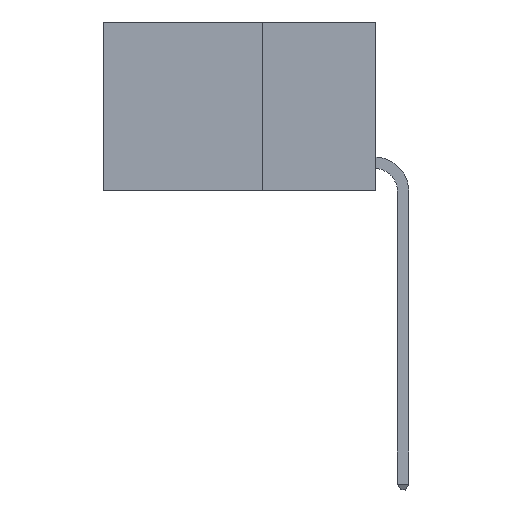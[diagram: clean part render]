
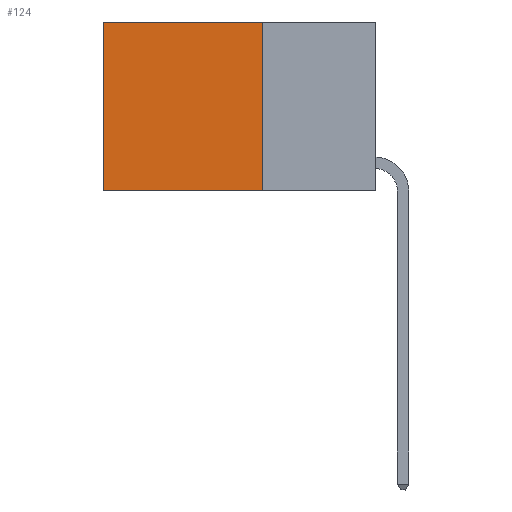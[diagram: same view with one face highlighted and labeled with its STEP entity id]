
A CAD part, left-side view. The second image highlights one B-rep face of the part: STEP entity #124.
In plain terms, the highlighted planar face has unit normal (-1, 0, 0).
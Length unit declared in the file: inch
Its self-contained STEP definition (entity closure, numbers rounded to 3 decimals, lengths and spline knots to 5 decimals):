
#124 = ADVANCED_FACE ( 'NONE', ( #5237 ), #10010, .F. ) ;
#267 = CARTESIAN_POINT ( 'NONE',  ( 0.2625, 0.25, 0. ) ) ;
#365 = EDGE_LOOP ( 'NONE', ( #4084, #5234, #2680, #2162 ) ) ;
#497 = AXIS2_PLACEMENT_3D ( 'NONE', #1657, #8894, #3595 ) ;
#1501 = EDGE_CURVE ( 'NONE', #4371, #6391, #4282, .T. ) ;
#1657 = CARTESIAN_POINT ( 'NONE',  ( 0.2625, 0.25, 0. ) ) ;
#1768 = LINE ( 'NONE', #4494, #8416 ) ;
#2078 = LINE ( 'NONE', #3456, #6371 ) ;
#2162 = ORIENTED_EDGE ( 'NONE', *, *, #1501, .T. ) ;
#2516 = VERTEX_POINT ( 'NONE', #8042 ) ;
#2680 = ORIENTED_EDGE ( 'NONE', *, *, #6763, .F. ) ;
#2996 = EDGE_CURVE ( 'NONE', #4859, #2516, #2078, .T. ) ;
#3369 = DIRECTION ( 'NONE',  ( 0., 1., 0. ) ) ;
#3456 = CARTESIAN_POINT ( 'NONE',  ( 0.2625, 0.25, -0.37 ) ) ;
#3595 = DIRECTION ( 'NONE',  ( 0., 0., -1. ) ) ;
#4008 = VECTOR ( 'NONE', #4724, 39.37008 ) ;
#4084 = ORIENTED_EDGE ( 'NONE', *, *, #8948, .T. ) ;
#4282 = LINE ( 'NONE', #4687, #4008 ) ;
#4371 = VERTEX_POINT ( 'NONE', #4455 ) ;
#4455 = CARTESIAN_POINT ( 'NONE',  ( 0.2625, 0.25, 0. ) ) ;
#4494 = CARTESIAN_POINT ( 'NONE',  ( 0.2625, 0.6, 0. ) ) ;
#4687 = CARTESIAN_POINT ( 'NONE',  ( 0.2625, 0.25, 0. ) ) ;
#4724 = DIRECTION ( 'NONE',  ( 0., 1., 0. ) ) ;
#4859 = VERTEX_POINT ( 'NONE', #5067 ) ;
#5067 = CARTESIAN_POINT ( 'NONE',  ( 0.2625, 0.25, -0.37 ) ) ;
#5234 = ORIENTED_EDGE ( 'NONE', *, *, #2996, .F. ) ;
#5237 = FACE_OUTER_BOUND ( 'NONE', #365, .T. ) ;
#5340 = DIRECTION ( 'NONE',  ( 0., 0., -1. ) ) ;
#6371 = VECTOR ( 'NONE', #3369, 39.37008 ) ;
#6391 = VERTEX_POINT ( 'NONE', #9317 ) ;
#6763 = EDGE_CURVE ( 'NONE', #4371, #4859, #10930, .T. ) ;
#8042 = CARTESIAN_POINT ( 'NONE',  ( 0.2625, 0.6, -0.37 ) ) ;
#8185 = DIRECTION ( 'NONE',  ( 0., 0., -1. ) ) ;
#8416 = VECTOR ( 'NONE', #5340, 39.37008 ) ;
#8894 = DIRECTION ( 'NONE',  ( 1., 0., 0. ) ) ;
#8948 = EDGE_CURVE ( 'NONE', #6391, #2516, #1768, .T. ) ;
#9317 = CARTESIAN_POINT ( 'NONE',  ( 0.2625, 0.6, 0. ) ) ;
#10010 = PLANE ( 'NONE',  #497 ) ;
#10422 = VECTOR ( 'NONE', #8185, 39.37008 ) ;
#10930 = LINE ( 'NONE', #267, #10422 ) ;
